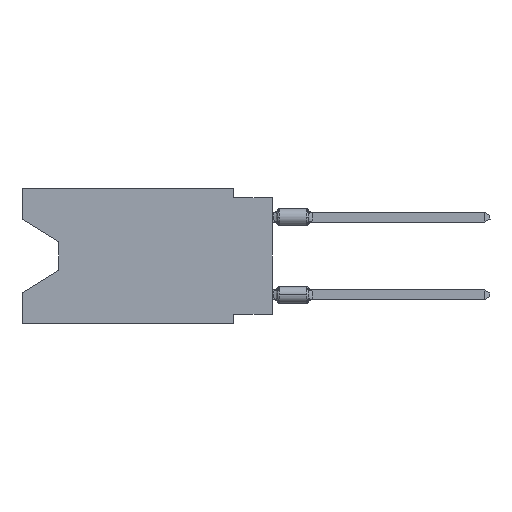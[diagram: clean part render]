
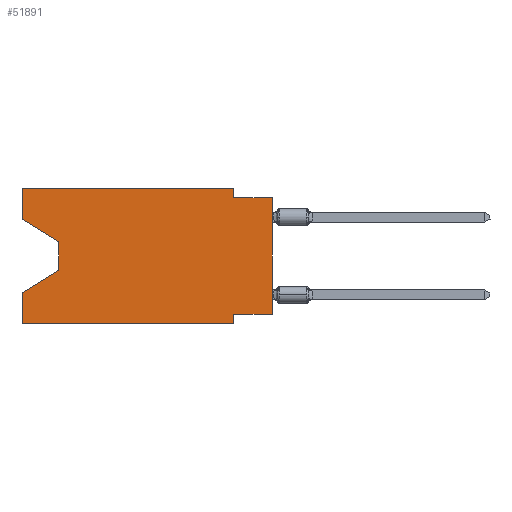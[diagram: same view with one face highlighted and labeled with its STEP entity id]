
A CAD part, left-side view. The second image highlights one B-rep face of the part: STEP entity #51891.
In plain terms, the highlighted planar face has unit normal (-1, 0, 0).
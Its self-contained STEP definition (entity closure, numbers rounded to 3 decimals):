
#186 = DIRECTION ( 'NONE',  ( 0., -1., 0. ) ) ;
#2201 = ORIENTED_EDGE ( 'NONE', *, *, #18321, .F. ) ;
#2532 = LINE ( 'NONE', #23731, #24335 ) ;
#2627 = CARTESIAN_POINT ( 'NONE',  ( 0., 0., -8.255 ) ) ;
#2956 = CARTESIAN_POINT ( 'NONE',  ( 0., 2.54, -8.255 ) ) ;
#3552 = CARTESIAN_POINT ( 'NONE',  ( 0., 16.383, -6.852 ) ) ;
#5865 = CARTESIAN_POINT ( 'NONE',  ( 0., 2.54, 0. ) ) ;
#5967 = EDGE_CURVE ( 'NONE', #39618, #46403, #2532, .T. ) ;
#6652 = VECTOR ( 'NONE', #31252, 1000. ) ;
#6793 = VECTOR ( 'NONE', #30615, 1000. ) ;
#7251 = VECTOR ( 'NONE', #53453, 1000. ) ;
#7616 = CARTESIAN_POINT ( 'NONE',  ( 0., 2.54, 0. ) ) ;
#7688 = VERTEX_POINT ( 'NONE', #3552 ) ;
#9106 = EDGE_CURVE ( 'NONE', #26502, #39618, #20747, .T. ) ;
#10317 = LINE ( 'NONE', #14655, #6652 ) ;
#11338 = ORIENTED_EDGE ( 'NONE', *, *, #46553, .F. ) ;
#11341 = CARTESIAN_POINT ( 'NONE',  ( 0., 13.97, -3.505 ) ) ;
#11435 = CARTESIAN_POINT ( 'NONE',  ( 0., 2.54, -0.635 ) ) ;
#11929 = PLANE ( 'NONE',  #36110 ) ;
#12119 = ORIENTED_EDGE ( 'NONE', *, *, #9106, .F. ) ;
#12918 = ORIENTED_EDGE ( 'NONE', *, *, #31074, .T. ) ;
#13370 = VERTEX_POINT ( 'NONE', #45705 ) ;
#14655 = CARTESIAN_POINT ( 'NONE',  ( 0., 13.97, -5.385 ) ) ;
#15375 = VERTEX_POINT ( 'NONE', #25594 ) ;
#17226 = CARTESIAN_POINT ( 'NONE',  ( 0., 16.383, -2.038 ) ) ;
#17319 = ORIENTED_EDGE ( 'NONE', *, *, #49290, .F. ) ;
#17581 = EDGE_CURVE ( 'NONE', #51853, #46403, #25714, .T. ) ;
#17792 = ORIENTED_EDGE ( 'NONE', *, *, #17581, .T. ) ;
#18321 = EDGE_CURVE ( 'NONE', #37068, #41767, #41848, .T. ) ;
#18644 = LINE ( 'NONE', #5865, #6793 ) ;
#18904 = VECTOR ( 'NONE', #44512, 1000. ) ;
#20747 = LINE ( 'NONE', #25621, #40317 ) ;
#21798 = ORIENTED_EDGE ( 'NONE', *, *, #26786, .F. ) ;
#21816 = EDGE_CURVE ( 'NONE', #13370, #30633, #48580, .T. ) ;
#22115 = EDGE_CURVE ( 'NONE', #42554, #37068, #18644, .T. ) ;
#22221 = LINE ( 'NONE', #45893, #27436 ) ;
#23272 = EDGE_LOOP ( 'NONE', ( #12918, #43597, #40548, #11338, #17792, #35036, #12119, #49288, #2201, #43516, #17319, #21798 ) ) ;
#23386 = DIRECTION ( 'NONE',  ( 0., 0., 1. ) ) ;
#23445 = CARTESIAN_POINT ( 'NONE',  ( 0., 0., -0.635 ) ) ;
#23731 = CARTESIAN_POINT ( 'NONE',  ( 0., 2.54, -8.89 ) ) ;
#24335 = VECTOR ( 'NONE', #32166, 1000. ) ;
#24433 = DIRECTION ( 'NONE',  ( 1., 0., 0. ) ) ;
#25330 = EDGE_CURVE ( 'NONE', #26502, #41767, #53520, .T. ) ;
#25354 = DIRECTION ( 'NONE',  ( 0., 1., 0. ) ) ;
#25594 = CARTESIAN_POINT ( 'NONE',  ( 0., 16.383, 0. ) ) ;
#25621 = CARTESIAN_POINT ( 'NONE',  ( 0., 0., -8.255 ) ) ;
#25714 = LINE ( 'NONE', #50436, #32519 ) ;
#26502 = VERTEX_POINT ( 'NONE', #2627 ) ;
#26786 = EDGE_CURVE ( 'NONE', #48549, #15375, #53170, .T. ) ;
#27265 = CARTESIAN_POINT ( 'NONE',  ( 0., 13.97, -5.385 ) ) ;
#27436 = VECTOR ( 'NONE', #41833, 1000. ) ;
#28455 = DIRECTION ( 'NONE',  ( 0., 0., 1. ) ) ;
#30615 = DIRECTION ( 'NONE',  ( 0., 0., -1. ) ) ;
#30633 = VERTEX_POINT ( 'NONE', #27265 ) ;
#30937 = CARTESIAN_POINT ( 'NONE',  ( 0., 2.54, -8.89 ) ) ;
#30957 = VECTOR ( 'NONE', #28455, 1000. ) ;
#31015 = CARTESIAN_POINT ( 'NONE',  ( 0., 16.383, -2.038 ) ) ;
#31074 = EDGE_CURVE ( 'NONE', #48549, #13370, #34563, .T. ) ;
#31252 = DIRECTION ( 'NONE',  ( 0., 0.855, -0.519 ) ) ;
#32166 = DIRECTION ( 'NONE',  ( 0., 0., -1. ) ) ;
#32519 = VECTOR ( 'NONE', #186, 1000. ) ;
#32540 = CARTESIAN_POINT ( 'NONE',  ( 0., 16.383, 0. ) ) ;
#34563 = LINE ( 'NONE', #31015, #50771 ) ;
#35036 = ORIENTED_EDGE ( 'NONE', *, *, #5967, .F. ) ;
#35086 = CARTESIAN_POINT ( 'NONE',  ( 0., 16.383, -8.89 ) ) ;
#36110 = AXIS2_PLACEMENT_3D ( 'NONE', #53243, #24433, #48896 ) ;
#37068 = VERTEX_POINT ( 'NONE', #11435 ) ;
#39618 = VERTEX_POINT ( 'NONE', #2956 ) ;
#39683 = EDGE_CURVE ( 'NONE', #30633, #7688, #10317, .T. ) ;
#40317 = VECTOR ( 'NONE', #25354, 1000. ) ;
#40548 = ORIENTED_EDGE ( 'NONE', *, *, #39683, .T. ) ;
#41661 = VECTOR ( 'NONE', #23386, 1000. ) ;
#41767 = VERTEX_POINT ( 'NONE', #51454 ) ;
#41833 = DIRECTION ( 'NONE',  ( 0., -1., 0. ) ) ;
#41848 = LINE ( 'NONE', #23445, #51647 ) ;
#42554 = VERTEX_POINT ( 'NONE', #7616 ) ;
#43516 = ORIENTED_EDGE ( 'NONE', *, *, #22115, .F. ) ;
#43597 = ORIENTED_EDGE ( 'NONE', *, *, #21816, .T. ) ;
#44285 = FACE_OUTER_BOUND ( 'NONE', #23272, .T. ) ;
#44512 = DIRECTION ( 'NONE',  ( 0., 0., -1. ) ) ;
#44774 = CARTESIAN_POINT ( 'NONE',  ( 0., 16.383, 0. ) ) ;
#45705 = CARTESIAN_POINT ( 'NONE',  ( 0., 13.97, -3.505 ) ) ;
#45893 = CARTESIAN_POINT ( 'NONE',  ( 0., 16.383, 0. ) ) ;
#46403 = VERTEX_POINT ( 'NONE', #30937 ) ;
#46553 = EDGE_CURVE ( 'NONE', #51853, #7688, #53187, .T. ) ;
#47584 = DIRECTION ( 'NONE',  ( 0., -0.855, -0.519 ) ) ;
#48163 = DIRECTION ( 'NONE',  ( 0., -1., 0. ) ) ;
#48549 = VERTEX_POINT ( 'NONE', #17226 ) ;
#48580 = LINE ( 'NONE', #11341, #18904 ) ;
#48896 = DIRECTION ( 'NONE',  ( 0., 0., -1. ) ) ;
#49288 = ORIENTED_EDGE ( 'NONE', *, *, #25330, .T. ) ;
#49290 = EDGE_CURVE ( 'NONE', #15375, #42554, #22221, .T. ) ;
#50436 = CARTESIAN_POINT ( 'NONE',  ( 0., 16.383, -8.89 ) ) ;
#50771 = VECTOR ( 'NONE', #47584, 1000. ) ;
#51454 = CARTESIAN_POINT ( 'NONE',  ( 0., 0., -0.635 ) ) ;
#51647 = VECTOR ( 'NONE', #48163, 1000. ) ;
#51853 = VERTEX_POINT ( 'NONE', #35086 ) ;
#51891 = ADVANCED_FACE ( 'NONE', ( #44285 ), #11929, .F. ) ;
#52717 = CARTESIAN_POINT ( 'NONE',  ( 0., 0., 0. ) ) ;
#53170 = LINE ( 'NONE', #32540, #30957 ) ;
#53187 = LINE ( 'NONE', #44774, #7251 ) ;
#53243 = CARTESIAN_POINT ( 'NONE',  ( 0., 16.383, 0. ) ) ;
#53453 = DIRECTION ( 'NONE',  ( 0., 0., 1. ) ) ;
#53520 = LINE ( 'NONE', #52717, #41661 ) ;
